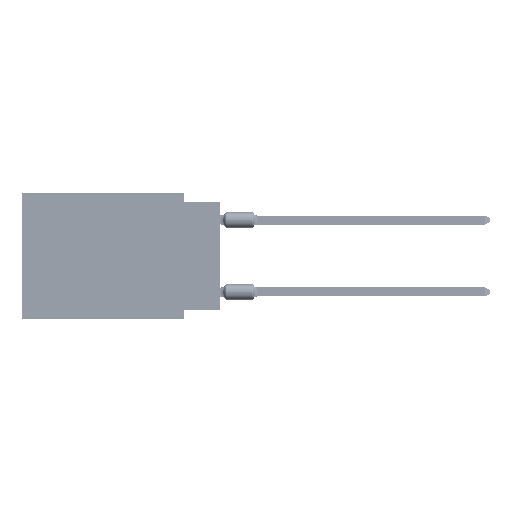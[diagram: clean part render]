
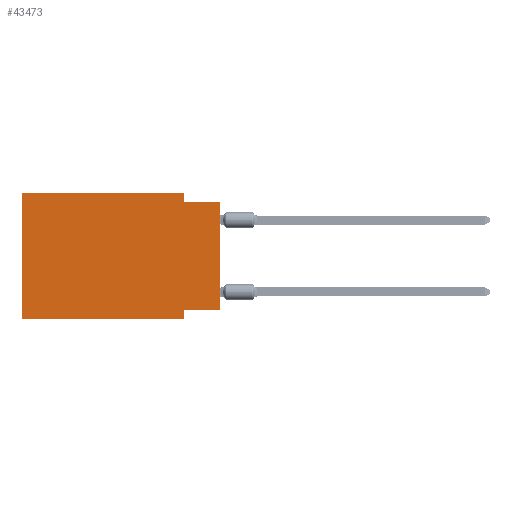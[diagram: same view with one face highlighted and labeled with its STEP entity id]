
A CAD part, left-side view. The second image highlights one B-rep face of the part: STEP entity #43473.
In plain terms, the highlighted planar face has unit normal (-1, 0, 0).
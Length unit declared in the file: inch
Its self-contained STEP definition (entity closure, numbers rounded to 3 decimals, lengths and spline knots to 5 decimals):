
#105 = DIRECTION ( 'NONE',  ( 1., 0., 0. ) ) ;
#574 = VECTOR ( 'NONE', #9469, 39.37008 ) ;
#4660 = CARTESIAN_POINT ( 'NONE',  ( 0., 0., -0.025 ) ) ;
#5100 = LINE ( 'NONE', #59056, #7086 ) ;
#7086 = VECTOR ( 'NONE', #20670, 39.37008 ) ;
#7445 = CARTESIAN_POINT ( 'NONE',  ( 0., 0.1, -0.35 ) ) ;
#9469 = DIRECTION ( 'NONE',  ( 0., 0., -1. ) ) ;
#9577 = DIRECTION ( 'NONE',  ( 0., 0., 1. ) ) ;
#10305 = VERTEX_POINT ( 'NONE', #29097 ) ;
#13763 = CARTESIAN_POINT ( 'NONE',  ( 0., 0.55, -0.35 ) ) ;
#14285 = ORIENTED_EDGE ( 'NONE', *, *, #63988, .F. ) ;
#14495 = CARTESIAN_POINT ( 'NONE',  ( 0., 0., -0.325 ) ) ;
#20135 = VERTEX_POINT ( 'NONE', #13763 ) ;
#20670 = DIRECTION ( 'NONE',  ( 0., -1., 0. ) ) ;
#23511 = EDGE_CURVE ( 'NONE', #27277, #64128, #64730, .T. ) ;
#27277 = VERTEX_POINT ( 'NONE', #78461 ) ;
#29097 = CARTESIAN_POINT ( 'NONE',  ( 0., 0.55, 0. ) ) ;
#31085 = DIRECTION ( 'NONE',  ( 0., 1., 0. ) ) ;
#31645 = EDGE_CURVE ( 'NONE', #81867, #77672, #34291, .T. ) ;
#32099 = CARTESIAN_POINT ( 'NONE',  ( 0., 0.1, -0.025 ) ) ;
#34291 = LINE ( 'NONE', #43937, #81376 ) ;
#34442 = FACE_OUTER_BOUND ( 'NONE', #55586, .T. ) ;
#34957 = EDGE_CURVE ( 'NONE', #81867, #42905, #71984, .T. ) ;
#36061 = ORIENTED_EDGE ( 'NONE', *, *, #55816, .F. ) ;
#36938 = DIRECTION ( 'NONE',  ( 0., -1., 0. ) ) ;
#37049 = DIRECTION ( 'NONE',  ( 0., 0., 1. ) ) ;
#37831 = VERTEX_POINT ( 'NONE', #57730 ) ;
#38528 = PLANE ( 'NONE',  #50142 ) ;
#38596 = VECTOR ( 'NONE', #9577, 39.37008 ) ;
#39832 = EDGE_CURVE ( 'NONE', #10305, #27277, #5100, .T. ) ;
#41479 = ORIENTED_EDGE ( 'NONE', *, *, #67798, .T. ) ;
#41766 = VECTOR ( 'NONE', #36938, 39.37008 ) ;
#42905 = VERTEX_POINT ( 'NONE', #71040 ) ;
#43473 = ADVANCED_FACE ( 'NONE', ( #34442 ), #38528, .F. ) ;
#43937 = CARTESIAN_POINT ( 'NONE',  ( 0., 0., -0.325 ) ) ;
#44948 = DIRECTION ( 'NONE',  ( 0., 0., -1. ) ) ;
#46139 = DIRECTION ( 'NONE',  ( 0., 0., -1. ) ) ;
#47878 = CARTESIAN_POINT ( 'NONE',  ( 0., 0.1, 0. ) ) ;
#47984 = CARTESIAN_POINT ( 'NONE',  ( 0., 0.55, 0. ) ) ;
#49054 = LINE ( 'NONE', #56954, #62053 ) ;
#49650 = CARTESIAN_POINT ( 'NONE',  ( 0., 0., 0. ) ) ;
#50142 = AXIS2_PLACEMENT_3D ( 'NONE', #76590, #105, #44948 ) ;
#54473 = EDGE_CURVE ( 'NONE', #20135, #10305, #68606, .T. ) ;
#54981 = VECTOR ( 'NONE', #37049, 39.37008 ) ;
#55586 = EDGE_LOOP ( 'NONE', ( #57039, #14285, #61522, #75156, #61572, #41479, #36061, #70119 ) ) ;
#55816 = EDGE_CURVE ( 'NONE', #77672, #37831, #77508, .T. ) ;
#56954 = CARTESIAN_POINT ( 'NONE',  ( 0., 0.55, -0.35 ) ) ;
#57039 = ORIENTED_EDGE ( 'NONE', *, *, #34957, .T. ) ;
#57730 = CARTESIAN_POINT ( 'NONE',  ( 0., 0.1, -0.35 ) ) ;
#59056 = CARTESIAN_POINT ( 'NONE',  ( 0., 0.55, 0. ) ) ;
#60491 = VECTOR ( 'NONE', #46139, 39.37008 ) ;
#60800 = LINE ( 'NONE', #4660, #41766 ) ;
#61522 = ORIENTED_EDGE ( 'NONE', *, *, #23511, .F. ) ;
#61572 = ORIENTED_EDGE ( 'NONE', *, *, #54473, .F. ) ;
#62053 = VECTOR ( 'NONE', #76261, 39.37008 ) ;
#63988 = EDGE_CURVE ( 'NONE', #64128, #42905, #60800, .T. ) ;
#64128 = VERTEX_POINT ( 'NONE', #32099 ) ;
#64730 = LINE ( 'NONE', #47878, #574 ) ;
#67798 = EDGE_CURVE ( 'NONE', #20135, #37831, #49054, .T. ) ;
#68606 = LINE ( 'NONE', #47984, #38596 ) ;
#68641 = CARTESIAN_POINT ( 'NONE',  ( 0., 0.1, -0.325 ) ) ;
#70119 = ORIENTED_EDGE ( 'NONE', *, *, #31645, .F. ) ;
#71040 = CARTESIAN_POINT ( 'NONE',  ( 0., 0., -0.025 ) ) ;
#71984 = LINE ( 'NONE', #49650, #54981 ) ;
#75156 = ORIENTED_EDGE ( 'NONE', *, *, #39832, .F. ) ;
#76261 = DIRECTION ( 'NONE',  ( 0., -1., 0. ) ) ;
#76590 = CARTESIAN_POINT ( 'NONE',  ( 0., 0.55, 0. ) ) ;
#77508 = LINE ( 'NONE', #7445, #60491 ) ;
#77672 = VERTEX_POINT ( 'NONE', #68641 ) ;
#78461 = CARTESIAN_POINT ( 'NONE',  ( 0., 0.1, 0. ) ) ;
#81376 = VECTOR ( 'NONE', #31085, 39.37008 ) ;
#81867 = VERTEX_POINT ( 'NONE', #14495 ) ;
